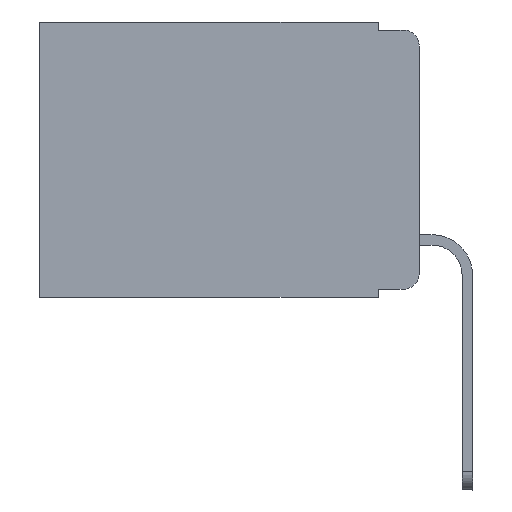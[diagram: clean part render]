
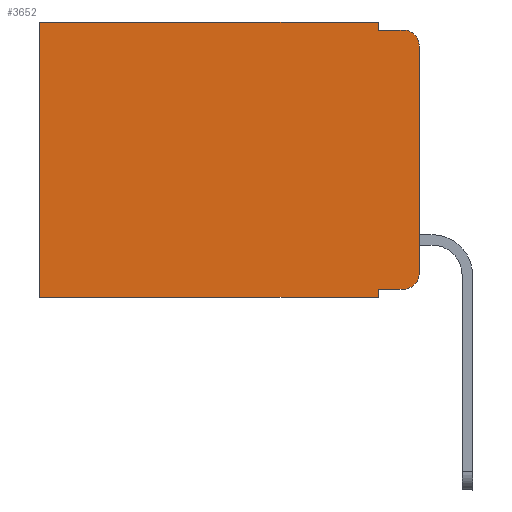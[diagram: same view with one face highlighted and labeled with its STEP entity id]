
A CAD part, left-side view. The second image highlights one B-rep face of the part: STEP entity #3652.
In plain terms, the highlighted planar face has unit normal (-1, 0, 0).
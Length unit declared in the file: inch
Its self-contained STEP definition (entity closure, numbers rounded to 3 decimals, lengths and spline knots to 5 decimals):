
#22 = CARTESIAN_POINT ( 'NONE',  ( 0.298, 0.02, -0.313 ) ) ;
#286 = LINE ( 'NONE', #2983, #10207 ) ;
#334 = VECTOR ( 'NONE', #4710, 39.37008 ) ;
#477 = LINE ( 'NONE', #10649, #4175 ) ;
#687 = LINE ( 'NONE', #1408, #3851 ) ;
#852 = LINE ( 'NONE', #1830, #878 ) ;
#878 = VECTOR ( 'NONE', #5021, 39.37008 ) ;
#975 = PLANE ( 'NONE',  #10102 ) ;
#1365 = LINE ( 'NONE', #5711, #334 ) ;
#1408 = CARTESIAN_POINT ( 'NONE',  ( 0.298, 0.051, 0. ) ) ;
#1544 = CARTESIAN_POINT ( 'NONE',  ( 0.298, 0.051, -0.01 ) ) ;
#1571 = ORIENTED_EDGE ( 'NONE', *, *, #7542, .T. ) ;
#1692 = DIRECTION ( 'NONE',  ( 0., 0., -1. ) ) ;
#1811 = ORIENTED_EDGE ( 'NONE', *, *, #2410, .T. ) ;
#1830 = CARTESIAN_POINT ( 'NONE',  ( 0.298, 0.051, -0.333 ) ) ;
#2036 = AXIS2_PLACEMENT_3D ( 'NONE', #22, #6353, #10520 ) ;
#2140 = EDGE_CURVE ( 'NONE', #6292, #5923, #9170, .T. ) ;
#2239 = EDGE_CURVE ( 'NONE', #3086, #8107, #3072, .T. ) ;
#2270 = VERTEX_POINT ( 'NONE', #9579 ) ;
#2294 = CARTESIAN_POINT ( 'NONE',  ( 0.298, 0.051, 0. ) ) ;
#2410 = EDGE_CURVE ( 'NONE', #4883, #10230, #9930, .T. ) ;
#2724 = DIRECTION ( 'NONE',  ( 0., 0., -1. ) ) ;
#2753 = VERTEX_POINT ( 'NONE', #6229 ) ;
#2844 = CARTESIAN_POINT ( 'NONE',  ( 0.298, 0.051, 0. ) ) ;
#2950 = CARTESIAN_POINT ( 'NONE',  ( 0.298, 0.473, 0. ) ) ;
#2983 = CARTESIAN_POINT ( 'NONE',  ( 0.298, 0., -0.343 ) ) ;
#3072 = CIRCLE ( 'NONE', #6607, 0.02 ) ;
#3086 = VERTEX_POINT ( 'NONE', #6662 ) ;
#3160 = DIRECTION ( 'NONE',  ( -1., 0., 0. ) ) ;
#3278 = EDGE_CURVE ( 'NONE', #5923, #8107, #7974, .T. ) ;
#3544 = VERTEX_POINT ( 'NONE', #8299 ) ;
#3595 = VECTOR ( 'NONE', #3730, 39.37008 ) ;
#3652 = ADVANCED_FACE ( 'NONE', ( #6044 ), #975, .F. ) ;
#3730 = DIRECTION ( 'NONE',  ( 0., -1., 0. ) ) ;
#3851 = VECTOR ( 'NONE', #9098, 39.37008 ) ;
#4175 = VECTOR ( 'NONE', #9001, 39.37008 ) ;
#4552 = VECTOR ( 'NONE', #10545, 39.37008 ) ;
#4710 = DIRECTION ( 'NONE',  ( 0., 0., -1. ) ) ;
#4883 = VERTEX_POINT ( 'NONE', #7482 ) ;
#4985 = ORIENTED_EDGE ( 'NONE', *, *, #6448, .T. ) ;
#5021 = DIRECTION ( 'NONE',  ( 0., -1., 0. ) ) ;
#5711 = CARTESIAN_POINT ( 'NONE',  ( 0.298, 0., 0. ) ) ;
#5923 = VERTEX_POINT ( 'NONE', #1544 ) ;
#6044 = FACE_OUTER_BOUND ( 'NONE', #8126, .T. ) ;
#6229 = CARTESIAN_POINT ( 'NONE',  ( 0.298, 0.051, -0.333 ) ) ;
#6259 = ORIENTED_EDGE ( 'NONE', *, *, #2239, .T. ) ;
#6292 = VERTEX_POINT ( 'NONE', #2844 ) ;
#6353 = DIRECTION ( 'NONE',  ( -1., 0., 0. ) ) ;
#6448 = EDGE_CURVE ( 'NONE', #6292, #2270, #477, .T. ) ;
#6541 = DIRECTION ( 'NONE',  ( 0., 0., -1. ) ) ;
#6607 = AXIS2_PLACEMENT_3D ( 'NONE', #10713, #3160, #6541 ) ;
#6662 = CARTESIAN_POINT ( 'NONE',  ( 0.298, 0., -0.03 ) ) ;
#7095 = CARTESIAN_POINT ( 'NONE',  ( 0.298, 0.02, -0.01 ) ) ;
#7181 = DIRECTION ( 'NONE',  ( 0., 1., 0. ) ) ;
#7482 = CARTESIAN_POINT ( 'NONE',  ( 0.298, 0.02, -0.333 ) ) ;
#7542 = EDGE_CURVE ( 'NONE', #2270, #3544, #7972, .T. ) ;
#7740 = DIRECTION ( 'NONE',  ( 1., 0., 0. ) ) ;
#7783 = ORIENTED_EDGE ( 'NONE', *, *, #9334, .F. ) ;
#7972 = LINE ( 'NONE', #2950, #4552 ) ;
#7974 = LINE ( 'NONE', #8900, #3595 ) ;
#8107 = VERTEX_POINT ( 'NONE', #7095 ) ;
#8126 = EDGE_LOOP ( 'NONE', ( #8831, #6259, #10131, #9020, #4985, #1571, #9428, #7783, #8901, #1811 ) ) ;
#8207 = EDGE_CURVE ( 'NONE', #2753, #4883, #852, .T. ) ;
#8299 = CARTESIAN_POINT ( 'NONE',  ( 0.298, 0.473, -0.343 ) ) ;
#8437 = CARTESIAN_POINT ( 'NONE',  ( 0.298, 0.051, -0.343 ) ) ;
#8831 = ORIENTED_EDGE ( 'NONE', *, *, #8914, .F. ) ;
#8900 = CARTESIAN_POINT ( 'NONE',  ( 0.298, 0.051, -0.01 ) ) ;
#8901 = ORIENTED_EDGE ( 'NONE', *, *, #8207, .T. ) ;
#8906 = CARTESIAN_POINT ( 'NONE',  ( 0.298, 0., -0.313 ) ) ;
#8914 = EDGE_CURVE ( 'NONE', #3086, #10230, #1365, .T. ) ;
#9001 = DIRECTION ( 'NONE',  ( 0., 1., 0. ) ) ;
#9020 = ORIENTED_EDGE ( 'NONE', *, *, #2140, .F. ) ;
#9098 = DIRECTION ( 'NONE',  ( 0., 0., -1. ) ) ;
#9170 = LINE ( 'NONE', #2294, #10632 ) ;
#9274 = CARTESIAN_POINT ( 'NONE',  ( 0.298, 0., 0. ) ) ;
#9334 = EDGE_CURVE ( 'NONE', #2753, #10771, #687, .T. ) ;
#9428 = ORIENTED_EDGE ( 'NONE', *, *, #10810, .F. ) ;
#9579 = CARTESIAN_POINT ( 'NONE',  ( 0.298, 0.473, 0. ) ) ;
#9930 = CIRCLE ( 'NONE', #2036, 0.02 ) ;
#10102 = AXIS2_PLACEMENT_3D ( 'NONE', #9274, #7740, #2724 ) ;
#10131 = ORIENTED_EDGE ( 'NONE', *, *, #3278, .F. ) ;
#10207 = VECTOR ( 'NONE', #7181, 39.37008 ) ;
#10230 = VERTEX_POINT ( 'NONE', #8906 ) ;
#10520 = DIRECTION ( 'NONE',  ( 0., 0., -1. ) ) ;
#10545 = DIRECTION ( 'NONE',  ( 0., 0., -1. ) ) ;
#10632 = VECTOR ( 'NONE', #1692, 39.37008 ) ;
#10649 = CARTESIAN_POINT ( 'NONE',  ( 0.298, 0., 0. ) ) ;
#10713 = CARTESIAN_POINT ( 'NONE',  ( 0.298, 0.02, -0.03 ) ) ;
#10771 = VERTEX_POINT ( 'NONE', #8437 ) ;
#10810 = EDGE_CURVE ( 'NONE', #10771, #3544, #286, .T. ) ;
